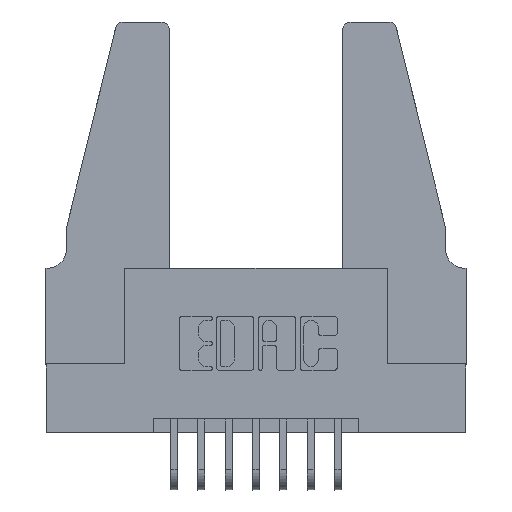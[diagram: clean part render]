
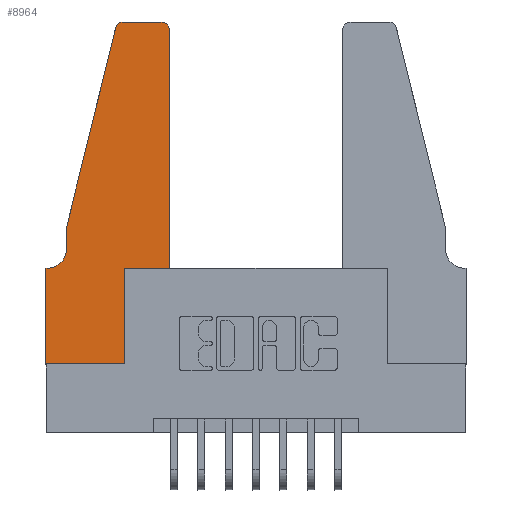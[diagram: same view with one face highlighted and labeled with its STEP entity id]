
A CAD part, top view. The second image highlights one B-rep face of the part: STEP entity #8964.
In plain terms, the highlighted planar face has unit normal (0, 0, 1).
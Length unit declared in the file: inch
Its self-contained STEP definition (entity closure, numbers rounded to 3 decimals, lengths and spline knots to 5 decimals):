
#190 = VERTEX_POINT ( 'NONE', #9802 ) ;
#370 = CARTESIAN_POINT ( 'NONE',  ( 0.0755, 0.5, 0.37 ) ) ;
#553 = CARTESIAN_POINT ( 'NONE',  ( 0.0755, 0.5, 0.37 ) ) ;
#664 = LINE ( 'NONE', #370, #8428 ) ;
#849 = CARTESIAN_POINT ( 'NONE',  ( 0., 0.35, 0.37 ) ) ;
#1277 = DIRECTION ( 'NONE',  ( 1., 0., 0. ) ) ;
#1281 = VECTOR ( 'NONE', #12492, 39.37008 ) ;
#1335 = EDGE_CURVE ( 'NONE', #7621, #5627, #664, .T. ) ;
#1352 = VECTOR ( 'NONE', #13847, 39.37008 ) ;
#1423 = AXIS2_PLACEMENT_3D ( 'NONE', #849, #9478, #12810 ) ;
#1590 = CARTESIAN_POINT ( 'NONE',  ( 0.2865, 0.35, 0.37 ) ) ;
#1731 = ORIENTED_EDGE ( 'NONE', *, *, #4208, .T. ) ;
#2595 = ORIENTED_EDGE ( 'NONE', *, *, #4318, .T. ) ;
#2706 = CARTESIAN_POINT ( 'NONE',  ( 0.0055, 0.42, 0.37 ) ) ;
#2734 = CARTESIAN_POINT ( 'NONE',  ( 0.0055, 0.35, 0.37 ) ) ;
#2762 = LINE ( 'NONE', #12501, #4106 ) ;
#2966 = EDGE_CURVE ( 'NONE', #7281, #8870, #10217, .T. ) ;
#2976 = CIRCLE ( 'NONE', #7821, 0.03 ) ;
#3089 = ORIENTED_EDGE ( 'NONE', *, *, #10932, .T. ) ;
#3102 = FACE_OUTER_BOUND ( 'NONE', #3895, .T. ) ;
#3519 = CARTESIAN_POINT ( 'NONE',  ( 0.4505, 0.35, 0.37 ) ) ;
#3520 = CARTESIAN_POINT ( 'NONE',  ( 0.4205, 1.25, 0.37 ) ) ;
#3782 = DIRECTION ( 'NONE',  ( -1., 0., 0. ) ) ;
#3799 = VECTOR ( 'NONE', #9718, 39.37008 ) ;
#3887 = VERTEX_POINT ( 'NONE', #5763 ) ;
#3895 = EDGE_LOOP ( 'NONE', ( #4002, #12355, #3089, #9293, #2595, #8703, #12034, #1731, #4754, #10010, #10403, #6637 ) ) ;
#3966 = LINE ( 'NONE', #8104, #1281 ) ;
#4002 = ORIENTED_EDGE ( 'NONE', *, *, #11634, .T. ) ;
#4068 = AXIS2_PLACEMENT_3D ( 'NONE', #2706, #10252, #3782 ) ;
#4106 = VECTOR ( 'NONE', #11442, 39.37008 ) ;
#4208 = EDGE_CURVE ( 'NONE', #3887, #5691, #11170, .T. ) ;
#4274 = EDGE_CURVE ( 'NONE', #7510, #190, #8826, .T. ) ;
#4318 = EDGE_CURVE ( 'NONE', #5627, #7510, #13904, .T. ) ;
#4415 = DIRECTION ( 'NONE',  ( 0., 0., 1. ) ) ;
#4597 = VECTOR ( 'NONE', #6135, 39.37008 ) ;
#4752 = CARTESIAN_POINT ( 'NONE',  ( 0.0755, 0.35, 0.37 ) ) ;
#4754 = ORIENTED_EDGE ( 'NONE', *, *, #12908, .T. ) ;
#4802 = DIRECTION ( 'NONE',  ( 0., 1., 0. ) ) ;
#4897 = VECTOR ( 'NONE', #10958, 39.37008 ) ;
#4913 = CARTESIAN_POINT ( 'NONE',  ( 0.2865, 0.35, 0.37 ) ) ;
#4935 = VERTEX_POINT ( 'NONE', #4913 ) ;
#5155 = PLANE ( 'NONE',  #1423 ) ;
#5627 = VERTEX_POINT ( 'NONE', #6322 ) ;
#5691 = VERTEX_POINT ( 'NONE', #8841 ) ;
#5696 = DIRECTION ( 'NONE',  ( 0., -1., 0. ) ) ;
#5763 = CARTESIAN_POINT ( 'NONE',  ( 0., 0., 0.37 ) ) ;
#5931 = EDGE_CURVE ( 'NONE', #4935, #7281, #8627, .T. ) ;
#6087 = CARTESIAN_POINT ( 'NONE',  ( 0.25487, 1.22718, 0.37 ) ) ;
#6135 = DIRECTION ( 'NONE',  ( -1., 0., 0. ) ) ;
#6322 = CARTESIAN_POINT ( 'NONE',  ( 0.0755, 0.42, 0.37 ) ) ;
#6637 = ORIENTED_EDGE ( 'NONE', *, *, #13765, .T. ) ;
#7281 = VERTEX_POINT ( 'NONE', #12644 ) ;
#7510 = VERTEX_POINT ( 'NONE', #2734 ) ;
#7614 = CARTESIAN_POINT ( 'NONE',  ( 0.284, 1.25, 0.37 ) ) ;
#7621 = VERTEX_POINT ( 'NONE', #553 ) ;
#7791 = VERTEX_POINT ( 'NONE', #6087 ) ;
#7821 = AXIS2_PLACEMENT_3D ( 'NONE', #11194, #10238, #13397 ) ;
#8104 = CARTESIAN_POINT ( 'NONE',  ( 0.0755, 0.5, 0.37 ) ) ;
#8428 = VECTOR ( 'NONE', #5696, 39.37008 ) ;
#8465 = VERTEX_POINT ( 'NONE', #7614 ) ;
#8627 = LINE ( 'NONE', #11832, #1352 ) ;
#8703 = ORIENTED_EDGE ( 'NONE', *, *, #4274, .T. ) ;
#8805 = CARTESIAN_POINT ( 'NONE',  ( 0., 0., 0.37 ) ) ;
#8826 = LINE ( 'NONE', #4752, #9509 ) ;
#8841 = CARTESIAN_POINT ( 'NONE',  ( 0.2865, 0., 0.37 ) ) ;
#8870 = VERTEX_POINT ( 'NONE', #10311 ) ;
#8964 = ADVANCED_FACE ( 'NONE', ( #3102 ), #5155, .T. ) ;
#8997 = VERTEX_POINT ( 'NONE', #3520 ) ;
#9097 = DIRECTION ( 'NONE',  ( -1., 0., 0. ) ) ;
#9293 = ORIENTED_EDGE ( 'NONE', *, *, #1335, .T. ) ;
#9478 = DIRECTION ( 'NONE',  ( 0., 0., 1. ) ) ;
#9509 = VECTOR ( 'NONE', #9097, 39.37008 ) ;
#9565 = CARTESIAN_POINT ( 'NONE',  ( 0.2605, 1.25, 0.37 ) ) ;
#9718 = DIRECTION ( 'NONE',  ( 0., 1., 0. ) ) ;
#9802 = CARTESIAN_POINT ( 'NONE',  ( 0., 0.35, 0.37 ) ) ;
#10010 = ORIENTED_EDGE ( 'NONE', *, *, #5931, .T. ) ;
#10217 = LINE ( 'NONE', #3519, #3799 ) ;
#10238 = DIRECTION ( 'NONE',  ( 0., 0., 1. ) ) ;
#10246 = EDGE_CURVE ( 'NONE', #8465, #7791, #2976, .T. ) ;
#10252 = DIRECTION ( 'NONE',  ( 0., 0., -1. ) ) ;
#10311 = CARTESIAN_POINT ( 'NONE',  ( 0.4505, 1.22, 0.37 ) ) ;
#10403 = ORIENTED_EDGE ( 'NONE', *, *, #2966, .T. ) ;
#10855 = AXIS2_PLACEMENT_3D ( 'NONE', #13205, #4415, #1277 ) ;
#10932 = EDGE_CURVE ( 'NONE', #7791, #7621, #3966, .T. ) ;
#10958 = DIRECTION ( 'NONE',  ( 1., 0., 0. ) ) ;
#11170 = LINE ( 'NONE', #8805, #4897 ) ;
#11181 = VECTOR ( 'NONE', #4802, 39.37008 ) ;
#11194 = CARTESIAN_POINT ( 'NONE',  ( 0.284, 1.22, 0.37 ) ) ;
#11442 = DIRECTION ( 'NONE',  ( 0., -1., 0. ) ) ;
#11634 = EDGE_CURVE ( 'NONE', #8997, #8465, #12431, .T. ) ;
#11832 = CARTESIAN_POINT ( 'NONE',  ( 0.4505, 0.35, 0.37 ) ) ;
#12034 = ORIENTED_EDGE ( 'NONE', *, *, #12120, .T. ) ;
#12120 = EDGE_CURVE ( 'NONE', #190, #3887, #2762, .T. ) ;
#12355 = ORIENTED_EDGE ( 'NONE', *, *, #10246, .T. ) ;
#12369 = CIRCLE ( 'NONE', #10855, 0.03 ) ;
#12431 = LINE ( 'NONE', #9565, #4597 ) ;
#12492 = DIRECTION ( 'NONE',  ( -0.239, -0.971, 0. ) ) ;
#12501 = CARTESIAN_POINT ( 'NONE',  ( 0., 0., 0.37 ) ) ;
#12568 = LINE ( 'NONE', #1590, #11181 ) ;
#12644 = CARTESIAN_POINT ( 'NONE',  ( 0.4505, 0.35, 0.37 ) ) ;
#12810 = DIRECTION ( 'NONE',  ( 1., 0., 0. ) ) ;
#12908 = EDGE_CURVE ( 'NONE', #5691, #4935, #12568, .T. ) ;
#13205 = CARTESIAN_POINT ( 'NONE',  ( 0.4205, 1.22, 0.37 ) ) ;
#13397 = DIRECTION ( 'NONE',  ( 1., 0., 0. ) ) ;
#13765 = EDGE_CURVE ( 'NONE', #8870, #8997, #12369, .T. ) ;
#13847 = DIRECTION ( 'NONE',  ( 1., 0., 0. ) ) ;
#13904 = CIRCLE ( 'NONE', #4068, 0.07 ) ;
